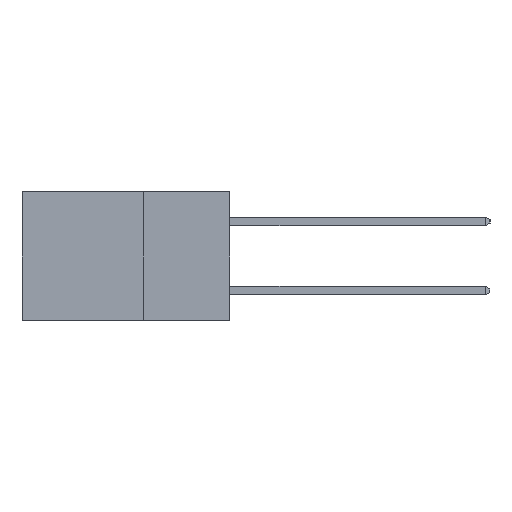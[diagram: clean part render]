
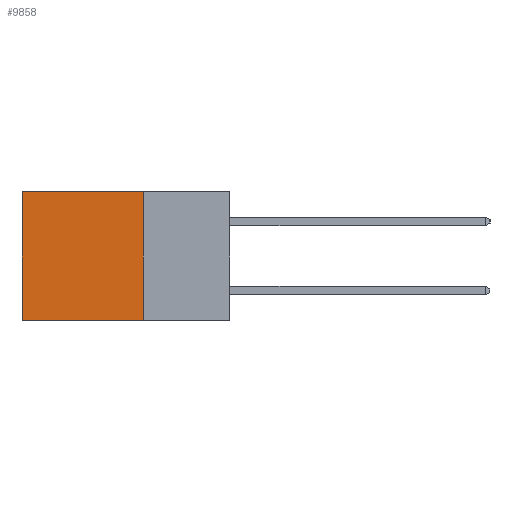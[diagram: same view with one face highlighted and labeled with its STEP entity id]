
A CAD part, left-side view. The second image highlights one B-rep face of the part: STEP entity #9858.
In plain terms, the highlighted planar face has unit normal (-1, 0, 0).
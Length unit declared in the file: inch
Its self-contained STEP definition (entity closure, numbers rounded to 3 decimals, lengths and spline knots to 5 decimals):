
#1682 = CARTESIAN_POINT ( 'NONE',  ( 0.2615, 0.25, -0.37 ) ) ;
#1778 = LINE ( 'NONE', #6360, #10072 ) ;
#2358 = FACE_OUTER_BOUND ( 'NONE', #7503, .T. ) ;
#2366 = ORIENTED_EDGE ( 'NONE', *, *, #9478, .T. ) ;
#3013 = AXIS2_PLACEMENT_3D ( 'NONE', #1682, #3473, #15797 ) ;
#3422 = VERTEX_POINT ( 'NONE', #22388 ) ;
#3473 = DIRECTION ( 'NONE',  ( 1., 0., 0. ) ) ;
#4022 = VERTEX_POINT ( 'NONE', #16941 ) ;
#4285 = EDGE_CURVE ( 'NONE', #3422, #7326, #7314, .T. ) ;
#4664 = DIRECTION ( 'NONE',  ( 0., 0., -1. ) ) ;
#4725 = CARTESIAN_POINT ( 'NONE',  ( 0.2615, 0.25, -0.37 ) ) ;
#5072 = EDGE_CURVE ( 'NONE', #5275, #4022, #13567, .T. ) ;
#5275 = VERTEX_POINT ( 'NONE', #4725 ) ;
#6140 = ORIENTED_EDGE ( 'NONE', *, *, #5072, .F. ) ;
#6360 = CARTESIAN_POINT ( 'NONE',  ( 0.2615, 0.25, -0.37 ) ) ;
#6778 = DIRECTION ( 'NONE',  ( 0., 1., 0. ) ) ;
#7064 = CARTESIAN_POINT ( 'NONE',  ( 0.2615, 0.25, -0.37 ) ) ;
#7314 = LINE ( 'NONE', #14230, #11974 ) ;
#7326 = VERTEX_POINT ( 'NONE', #16219 ) ;
#7503 = EDGE_LOOP ( 'NONE', ( #2366, #6140, #11423, #12764 ) ) ;
#7750 = DIRECTION ( 'NONE',  ( 0., 0., -1. ) ) ;
#8918 = VECTOR ( 'NONE', #6778, 39.37008 ) ;
#9478 = EDGE_CURVE ( 'NONE', #7326, #4022, #13951, .T. ) ;
#9853 = VECTOR ( 'NONE', #7750, 39.37008 ) ;
#9858 = ADVANCED_FACE ( 'NONE', ( #2358 ), #19186, .F. ) ;
#10072 = VECTOR ( 'NONE', #4664, 39.37008 ) ;
#11423 = ORIENTED_EDGE ( 'NONE', *, *, #15963, .F. ) ;
#11974 = VECTOR ( 'NONE', #14309, 39.37008 ) ;
#12764 = ORIENTED_EDGE ( 'NONE', *, *, #4285, .T. ) ;
#12959 = CARTESIAN_POINT ( 'NONE',  ( 0.2615, 0.6, -0.37 ) ) ;
#13567 = LINE ( 'NONE', #7064, #8918 ) ;
#13951 = LINE ( 'NONE', #12959, #9853 ) ;
#14230 = CARTESIAN_POINT ( 'NONE',  ( 0.2615, 0.25, 0. ) ) ;
#14309 = DIRECTION ( 'NONE',  ( 0., 1., 0. ) ) ;
#15797 = DIRECTION ( 'NONE',  ( 0., 0., -1. ) ) ;
#15963 = EDGE_CURVE ( 'NONE', #3422, #5275, #1778, .T. ) ;
#16219 = CARTESIAN_POINT ( 'NONE',  ( 0.2615, 0.6, 0. ) ) ;
#16941 = CARTESIAN_POINT ( 'NONE',  ( 0.2615, 0.6, -0.37 ) ) ;
#19186 = PLANE ( 'NONE',  #3013 ) ;
#22388 = CARTESIAN_POINT ( 'NONE',  ( 0.2615, 0.25, 0. ) ) ;
